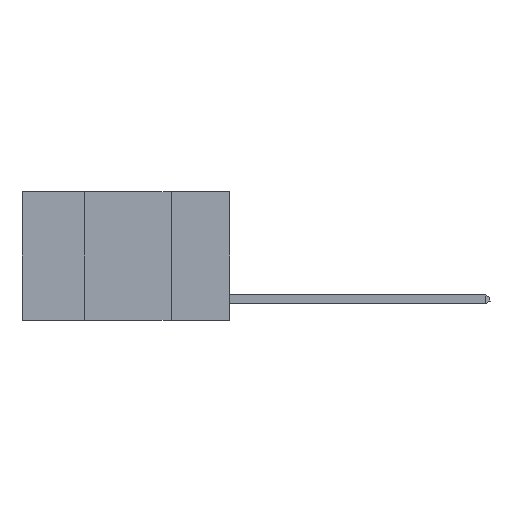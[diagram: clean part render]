
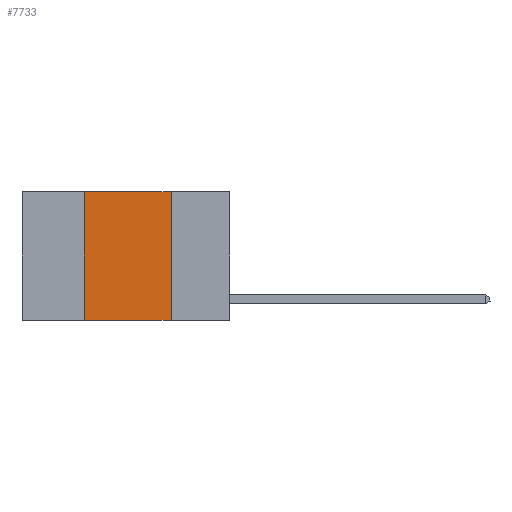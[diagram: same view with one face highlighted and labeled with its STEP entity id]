
A CAD part, left-side view. The second image highlights one B-rep face of the part: STEP entity #7733.
In plain terms, the highlighted planar face has unit normal (-1, 0, 0).
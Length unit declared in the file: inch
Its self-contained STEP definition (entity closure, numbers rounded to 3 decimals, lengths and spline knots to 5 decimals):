
#167 = VECTOR ( 'NONE', #5400, 39.37008 ) ;
#444 = CARTESIAN_POINT ( 'NONE',  ( 0., 0.42, 0. ) ) ;
#722 = ORIENTED_EDGE ( 'NONE', *, *, #5875, .F. ) ;
#798 = CARTESIAN_POINT ( 'NONE',  ( 0., 0.17, 0. ) ) ;
#1089 = AXIS2_PLACEMENT_3D ( 'NONE', #13634, #8232, #3799 ) ;
#1450 = ORIENTED_EDGE ( 'NONE', *, *, #11763, .T. ) ;
#2122 = ORIENTED_EDGE ( 'NONE', *, *, #8864, .F. ) ;
#2502 = CARTESIAN_POINT ( 'NONE',  ( 0., 0.42, 0. ) ) ;
#3137 = CARTESIAN_POINT ( 'NONE',  ( 0., 0.6, -0.37 ) ) ;
#3751 = VECTOR ( 'NONE', #11048, 39.37008 ) ;
#3799 = DIRECTION ( 'NONE',  ( 0., 0., -1. ) ) ;
#3926 = CARTESIAN_POINT ( 'NONE',  ( 0., 0.17, 0. ) ) ;
#4133 = LINE ( 'NONE', #10039, #167 ) ;
#4299 = CARTESIAN_POINT ( 'NONE',  ( 0., 0.17, -0.37 ) ) ;
#4670 = VECTOR ( 'NONE', #12469, 39.37008 ) ;
#4745 = EDGE_LOOP ( 'NONE', ( #2122, #13319, #722, #1450 ) ) ;
#5030 = DIRECTION ( 'NONE',  ( 0., 0., -1. ) ) ;
#5235 = VERTEX_POINT ( 'NONE', #798 ) ;
#5319 = LINE ( 'NONE', #3137, #3751 ) ;
#5400 = DIRECTION ( 'NONE',  ( 0., -1., 0. ) ) ;
#5807 = VERTEX_POINT ( 'NONE', #444 ) ;
#5875 = EDGE_CURVE ( 'NONE', #8467, #5807, #7287, .T. ) ;
#5949 = PLANE ( 'NONE',  #1089 ) ;
#7287 = LINE ( 'NONE', #2502, #4670 ) ;
#7733 = ADVANCED_FACE ( 'NONE', ( #12182 ), #5949, .F. ) ;
#8232 = DIRECTION ( 'NONE',  ( 1., 0., 0. ) ) ;
#8467 = VERTEX_POINT ( 'NONE', #12978 ) ;
#8864 = EDGE_CURVE ( 'NONE', #5235, #10864, #9921, .T. ) ;
#9407 = VECTOR ( 'NONE', #5030, 39.37008 ) ;
#9921 = LINE ( 'NONE', #3926, #9407 ) ;
#10039 = CARTESIAN_POINT ( 'NONE',  ( 0., 0.6, 0. ) ) ;
#10864 = VERTEX_POINT ( 'NONE', #4299 ) ;
#11048 = DIRECTION ( 'NONE',  ( 0., -1., 0. ) ) ;
#11763 = EDGE_CURVE ( 'NONE', #8467, #10864, #5319, .T. ) ;
#12182 = FACE_OUTER_BOUND ( 'NONE', #4745, .T. ) ;
#12274 = EDGE_CURVE ( 'NONE', #5807, #5235, #4133, .T. ) ;
#12469 = DIRECTION ( 'NONE',  ( 0., 0., 1. ) ) ;
#12978 = CARTESIAN_POINT ( 'NONE',  ( 0., 0.42, -0.37 ) ) ;
#13319 = ORIENTED_EDGE ( 'NONE', *, *, #12274, .F. ) ;
#13634 = CARTESIAN_POINT ( 'NONE',  ( 0., 0.6, 0. ) ) ;
